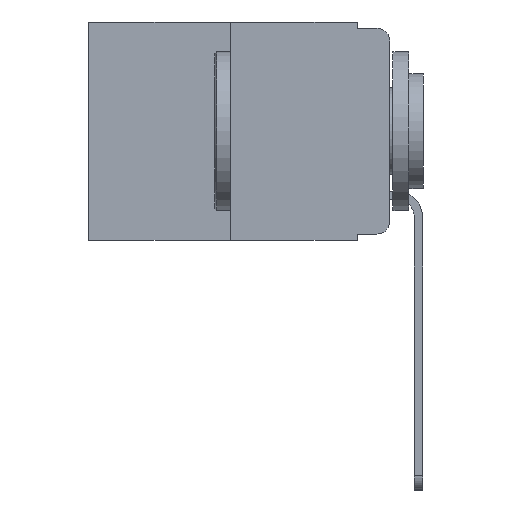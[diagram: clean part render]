
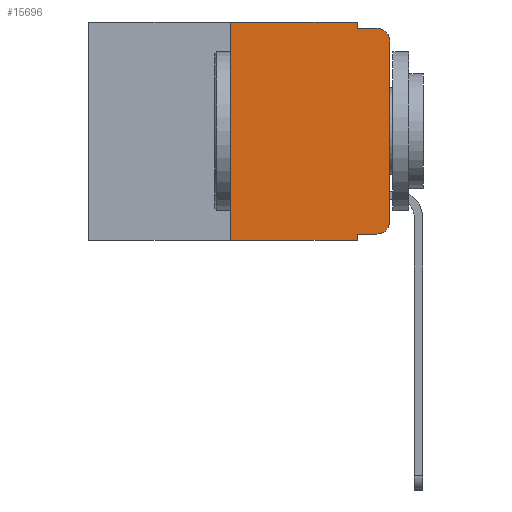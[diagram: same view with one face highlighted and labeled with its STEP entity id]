
A CAD part, left-side view. The second image highlights one B-rep face of the part: STEP entity #15696.
In plain terms, the highlighted planar face has unit normal (-1, 0, 0).
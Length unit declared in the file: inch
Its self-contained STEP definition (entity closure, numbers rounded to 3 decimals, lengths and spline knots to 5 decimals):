
#20 = DIRECTION ( 'NONE',  ( 0., -1., 0. ) ) ;
#288 = CARTESIAN_POINT ( 'NONE',  ( 0., 0.02, -0.01 ) ) ;
#920 = AXIS2_PLACEMENT_3D ( 'NONE', #15163, #7746, #8892 ) ;
#1358 = VERTEX_POINT ( 'NONE', #12690 ) ;
#1453 = ORIENTED_EDGE ( 'NONE', *, *, #9833, .F. ) ;
#1492 = ORIENTED_EDGE ( 'NONE', *, *, #4701, .F. ) ;
#1557 = CARTESIAN_POINT ( 'NONE',  ( 0., 0.02, -0.313 ) ) ;
#1785 = DIRECTION ( 'NONE',  ( 0., 0., 1. ) ) ;
#1993 = ORIENTED_EDGE ( 'NONE', *, *, #10370, .T. ) ;
#2036 = CARTESIAN_POINT ( 'NONE',  ( 0., 0., -0.03 ) ) ;
#2319 = LINE ( 'NONE', #12873, #12882 ) ;
#3065 = VECTOR ( 'NONE', #5692, 39.37008 ) ;
#3163 = DIRECTION ( 'NONE',  ( 0., 0., 1. ) ) ;
#3294 = LINE ( 'NONE', #9360, #4652 ) ;
#3694 = CARTESIAN_POINT ( 'NONE',  ( 0., 0.02, -0.03 ) ) ;
#3750 = EDGE_CURVE ( 'NONE', #11811, #14391, #9511, .T. ) ;
#3765 = AXIS2_PLACEMENT_3D ( 'NONE', #3694, #8421, #12137 ) ;
#3844 = VERTEX_POINT ( 'NONE', #15487 ) ;
#3863 = VERTEX_POINT ( 'NONE', #8117 ) ;
#4042 = DIRECTION ( 'NONE',  ( 0., 0., -1. ) ) ;
#4100 = EDGE_CURVE ( 'NONE', #1358, #15756, #14515, .T. ) ;
#4422 = VERTEX_POINT ( 'NONE', #2036 ) ;
#4652 = VECTOR ( 'NONE', #12575, 39.37008 ) ;
#4701 = EDGE_CURVE ( 'NONE', #11266, #3844, #7543, .T. ) ;
#4742 = EDGE_CURVE ( 'NONE', #11811, #3844, #14870, .T. ) ;
#5263 = DIRECTION ( 'NONE',  ( 0., -1., 0. ) ) ;
#5640 = VECTOR ( 'NONE', #20, 39.37008 ) ;
#5692 = DIRECTION ( 'NONE',  ( 0., 0., -1. ) ) ;
#6482 = VECTOR ( 'NONE', #15793, 39.37008 ) ;
#6592 = EDGE_CURVE ( 'NONE', #15756, #4422, #2319, .T. ) ;
#6919 = CARTESIAN_POINT ( 'NONE',  ( 0., 0.25, -0.343 ) ) ;
#7534 = CARTESIAN_POINT ( 'NONE',  ( 0., 0.25, 0. ) ) ;
#7543 = LINE ( 'NONE', #14999, #15621 ) ;
#7734 = ORIENTED_EDGE ( 'NONE', *, *, #4742, .T. ) ;
#7746 = DIRECTION ( 'NONE',  ( 1., 0., 0. ) ) ;
#8087 = EDGE_CURVE ( 'NONE', #14391, #15029, #3294, .T. ) ;
#8117 = CARTESIAN_POINT ( 'NONE',  ( 0., 0.051, -0.01 ) ) ;
#8383 = CARTESIAN_POINT ( 'NONE',  ( 0., 0.051, -0.01 ) ) ;
#8421 = DIRECTION ( 'NONE',  ( -1., 0., 0. ) ) ;
#8474 = CARTESIAN_POINT ( 'NONE',  ( 0., 0.051, -0.333 ) ) ;
#8824 = DIRECTION ( 'NONE',  ( 0., 0., -1. ) ) ;
#8892 = DIRECTION ( 'NONE',  ( 0., 0., -1. ) ) ;
#8916 = CARTESIAN_POINT ( 'NONE',  ( 0., 0.051, 0. ) ) ;
#8996 = EDGE_CURVE ( 'NONE', #15029, #3863, #10364, .T. ) ;
#9092 = ORIENTED_EDGE ( 'NONE', *, *, #12607, .T. ) ;
#9327 = FACE_OUTER_BOUND ( 'NONE', #10518, .T. ) ;
#9360 = CARTESIAN_POINT ( 'NONE',  ( 0., 0.473, 0. ) ) ;
#9504 = LINE ( 'NONE', #12267, #5640 ) ;
#9511 = LINE ( 'NONE', #11619, #10468 ) ;
#9833 = EDGE_CURVE ( 'NONE', #3863, #12081, #11700, .T. ) ;
#9991 = ORIENTED_EDGE ( 'NONE', *, *, #6592, .T. ) ;
#10242 = VECTOR ( 'NONE', #5263, 39.37008 ) ;
#10364 = LINE ( 'NONE', #10658, #3065 ) ;
#10370 = EDGE_CURVE ( 'NONE', #4422, #12081, #14962, .T. ) ;
#10468 = VECTOR ( 'NONE', #1785, 39.37008 ) ;
#10518 = EDGE_LOOP ( 'NONE', ( #9991, #1993, #1453, #13796, #12299, #12417, #7734, #1492, #9092, #13698 ) ) ;
#10658 = CARTESIAN_POINT ( 'NONE',  ( 0., 0.051, 0. ) ) ;
#10905 = AXIS2_PLACEMENT_3D ( 'NONE', #1557, #11498, #4042 ) ;
#11266 = VERTEX_POINT ( 'NONE', #8474 ) ;
#11498 = DIRECTION ( 'NONE',  ( -1., 0., 0. ) ) ;
#11511 = CARTESIAN_POINT ( 'NONE',  ( 0., 0., -0.313 ) ) ;
#11619 = CARTESIAN_POINT ( 'NONE',  ( 0., 0.25, 0. ) ) ;
#11700 = LINE ( 'NONE', #8383, #6482 ) ;
#11811 = VERTEX_POINT ( 'NONE', #6919 ) ;
#12081 = VERTEX_POINT ( 'NONE', #288 ) ;
#12137 = DIRECTION ( 'NONE',  ( 0., 0., -1. ) ) ;
#12267 = CARTESIAN_POINT ( 'NONE',  ( 0., 0.051, -0.333 ) ) ;
#12299 = ORIENTED_EDGE ( 'NONE', *, *, #8087, .F. ) ;
#12417 = ORIENTED_EDGE ( 'NONE', *, *, #3750, .F. ) ;
#12575 = DIRECTION ( 'NONE',  ( 0., -1., 0. ) ) ;
#12607 = EDGE_CURVE ( 'NONE', #11266, #1358, #9504, .T. ) ;
#12690 = CARTESIAN_POINT ( 'NONE',  ( 0., 0.02, -0.333 ) ) ;
#12873 = CARTESIAN_POINT ( 'NONE',  ( 0., 0., 0. ) ) ;
#12882 = VECTOR ( 'NONE', #3163, 39.37008 ) ;
#13698 = ORIENTED_EDGE ( 'NONE', *, *, #4100, .T. ) ;
#13796 = ORIENTED_EDGE ( 'NONE', *, *, #8996, .F. ) ;
#13937 = PLANE ( 'NONE',  #920 ) ;
#14391 = VERTEX_POINT ( 'NONE', #7534 ) ;
#14515 = CIRCLE ( 'NONE', #10905, 0.02 ) ;
#14870 = LINE ( 'NONE', #15141, #10242 ) ;
#14962 = CIRCLE ( 'NONE', #3765, 0.02 ) ;
#14999 = CARTESIAN_POINT ( 'NONE',  ( 0., 0.051, 0. ) ) ;
#15029 = VERTEX_POINT ( 'NONE', #8916 ) ;
#15141 = CARTESIAN_POINT ( 'NONE',  ( 0., 0.473, -0.343 ) ) ;
#15163 = CARTESIAN_POINT ( 'NONE',  ( 0., 0.473, 0. ) ) ;
#15487 = CARTESIAN_POINT ( 'NONE',  ( 0., 0.051, -0.343 ) ) ;
#15621 = VECTOR ( 'NONE', #8824, 39.37008 ) ;
#15696 = ADVANCED_FACE ( 'NONE', ( #9327 ), #13937, .F. ) ;
#15756 = VERTEX_POINT ( 'NONE', #11511 ) ;
#15793 = DIRECTION ( 'NONE',  ( 0., -1., 0. ) ) ;
